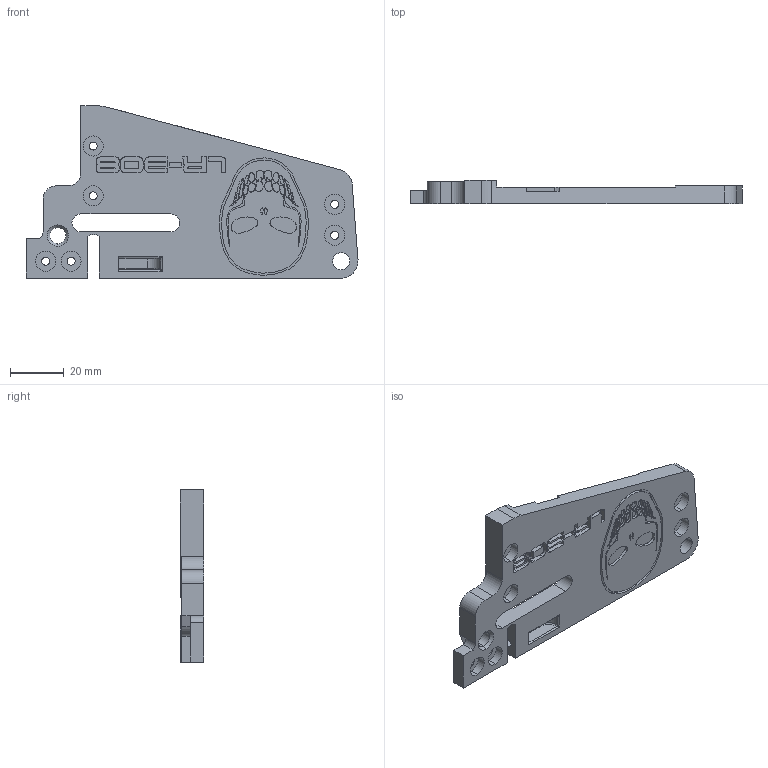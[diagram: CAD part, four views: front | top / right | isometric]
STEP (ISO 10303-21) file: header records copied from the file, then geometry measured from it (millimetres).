
FILE_DESCRIPTION (( 'STEP AP214' ), '1' );
FILE_NAME ('Thunderbolt_Mag_Well_Left.STEP', '2021-09-12T03:30:13', ( '' ), ( '' ), 'SwSTEP 2.0', 'SolidWorks 2020', '' );
FILE_SCHEMA (( 'AUTOMOTIVE_DESIGN' ));
Length unit declared in the file: millimetre
Products named in the file (1): Thunderbolt_Mag_Well_Left
Bounding box: 124.06 x 8.75 x 64.36 mm (x, y, z)
Volume: 34238.9 mm3; surface area: 16922.9 mm2
Topology: 1 solids, 1 shells, 296 faces, 728 edges, 471 vertices
Faces by surface type: plane 139, bspline 93, cylinder 57, sphere 3, cone 2, torus 2
Entity records: 12524 total; most frequent: CARTESIAN_POINT 6087, ORIENTED_EDGE 1446, DIRECTION 1038, EDGE_CURVE 723, VERTEX_POINT 471, LINE 418, VECTOR 418, EDGE_LOOP 358
